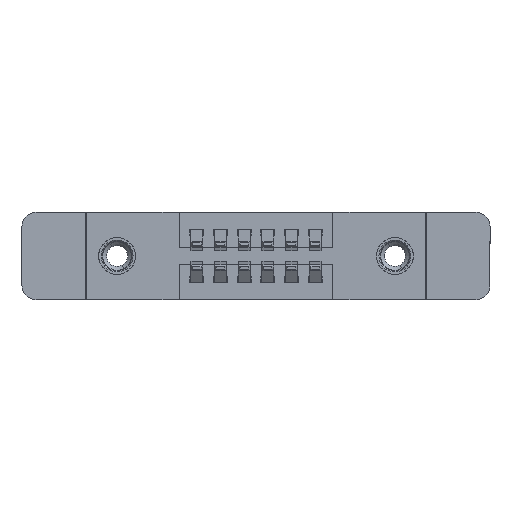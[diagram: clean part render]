
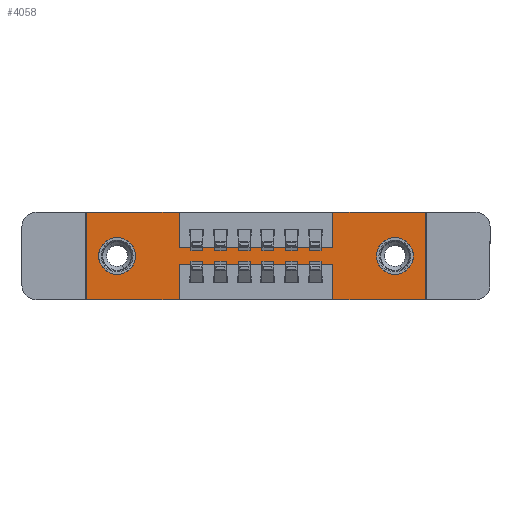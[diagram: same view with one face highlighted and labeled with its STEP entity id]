
A CAD part, front view. The second image highlights one B-rep face of the part: STEP entity #4058.
In plain terms, the highlighted planar face has unit normal (0, -1, 0).
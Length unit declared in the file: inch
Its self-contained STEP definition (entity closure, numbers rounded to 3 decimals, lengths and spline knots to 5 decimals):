
#70 = VECTOR ( 'NONE', #12861, 39.37008 ) ;
#97 = DIRECTION ( 'NONE',  ( 1., 0., 0. ) ) ;
#251 = VECTOR ( 'NONE', #13630, 39.37008 ) ;
#335 = CARTESIAN_POINT ( 'NONE',  ( 0.3925, 0., -0.22 ) ) ;
#415 = CARTESIAN_POINT ( 'NONE',  ( 0., 0., -0.37 ) ) ;
#432 = EDGE_CURVE ( 'NONE', #12691, #13546, #6473, .T. ) ;
#435 = CARTESIAN_POINT ( 'NONE',  ( 1.305, 0., -0.185 ) ) ;
#496 = VERTEX_POINT ( 'NONE', #5100 ) ;
#497 = VERTEX_POINT ( 'NONE', #13150 ) ;
#561 = VECTOR ( 'NONE', #97, 39.37008 ) ;
#679 = ORIENTED_EDGE ( 'NONE', *, *, #7101, .F. ) ;
#723 = ORIENTED_EDGE ( 'NONE', *, *, #10206, .T. ) ;
#831 = CARTESIAN_POINT ( 'NONE',  ( 1.0425, 0., -0.15 ) ) ;
#891 = CIRCLE ( 'NONE', #4677, 0.078 ) ;
#1075 = VECTOR ( 'NONE', #12570, 39.37008 ) ;
#1166 = CARTESIAN_POINT ( 'NONE',  ( 0.3925, 0., -0.15 ) ) ;
#1195 = DIRECTION ( 'NONE',  ( 0., 0., 1. ) ) ;
#1584 = DIRECTION ( 'NONE',  ( 0., 0., -1. ) ) ;
#1616 = DIRECTION ( 'NONE',  ( 0., 0., -1. ) ) ;
#1622 = CARTESIAN_POINT ( 'NONE',  ( 0.3925, 0., -0.15 ) ) ;
#1876 = VECTOR ( 'NONE', #10326, 39.37008 ) ;
#1908 = VERTEX_POINT ( 'NONE', #4619 ) ;
#2002 = ORIENTED_EDGE ( 'NONE', *, *, #9250, .F. ) ;
#2432 = AXIS2_PLACEMENT_3D ( 'NONE', #13286, #6387, #14426 ) ;
#2614 = LINE ( 'NONE', #8051, #5289 ) ;
#2642 = ORIENTED_EDGE ( 'NONE', *, *, #4196, .F. ) ;
#2768 = AXIS2_PLACEMENT_3D ( 'NONE', #435, #8440, #1584 ) ;
#3046 = LINE ( 'NONE', #7247, #8759 ) ;
#3229 = LINE ( 'NONE', #12070, #12024 ) ;
#3339 = CARTESIAN_POINT ( 'NONE',  ( 0., 0., 0. ) ) ;
#3596 = CARTESIAN_POINT ( 'NONE',  ( 1.0425, 0., -0.37 ) ) ;
#3885 = DIRECTION ( 'NONE',  ( -1., 0., 0. ) ) ;
#4048 = VERTEX_POINT ( 'NONE', #4407 ) ;
#4054 = ORIENTED_EDGE ( 'NONE', *, *, #432, .F. ) ;
#4058 = ADVANCED_FACE ( 'NONE', ( #5387, #14192, #11154 ), #12436, .T. ) ;
#4145 = LINE ( 'NONE', #11419, #1075 ) ;
#4196 = EDGE_CURVE ( 'NONE', #5480, #497, #6622, .T. ) ;
#4407 = CARTESIAN_POINT ( 'NONE',  ( 0.3925, 0., -0.22 ) ) ;
#4479 = EDGE_LOOP ( 'NONE', ( #13701, #4687 ) ) ;
#4540 = ORIENTED_EDGE ( 'NONE', *, *, #13030, .F. ) ;
#4611 = VERTEX_POINT ( 'NONE', #6480 ) ;
#4619 = CARTESIAN_POINT ( 'NONE',  ( 0., 0., -0.37 ) ) ;
#4648 = CARTESIAN_POINT ( 'NONE',  ( 0., 0., 0. ) ) ;
#4677 = AXIS2_PLACEMENT_3D ( 'NONE', #13163, #6266, #14307 ) ;
#4687 = ORIENTED_EDGE ( 'NONE', *, *, #11195, .T. ) ;
#4732 = DIRECTION ( 'NONE',  ( 0., 0., 1. ) ) ;
#4754 = CIRCLE ( 'NONE', #2432, 0.078 ) ;
#4905 = LINE ( 'NONE', #12632, #1876 ) ;
#4913 = ORIENTED_EDGE ( 'NONE', *, *, #11304, .F. ) ;
#5100 = CARTESIAN_POINT ( 'NONE',  ( 1.305, 0., -0.263 ) ) ;
#5289 = VECTOR ( 'NONE', #1195, 39.37008 ) ;
#5387 = FACE_BOUND ( 'NONE', #6741, .T. ) ;
#5480 = VERTEX_POINT ( 'NONE', #9616 ) ;
#5573 = CARTESIAN_POINT ( 'NONE',  ( 0., 0., -0.37 ) ) ;
#5585 = DIRECTION ( 'NONE',  ( 0., 1., 0. ) ) ;
#5994 = CARTESIAN_POINT ( 'NONE',  ( 0.13, 0., -0.107 ) ) ;
#6049 = CARTESIAN_POINT ( 'NONE',  ( 1.0425, 0., -0.37 ) ) ;
#6249 = VERTEX_POINT ( 'NONE', #7646 ) ;
#6266 = DIRECTION ( 'NONE',  ( 0., 1., 0. ) ) ;
#6321 = LINE ( 'NONE', #5573, #251 ) ;
#6387 = DIRECTION ( 'NONE',  ( 0., 1., 0. ) ) ;
#6451 = EDGE_LOOP ( 'NONE', ( #7751, #4540, #11044, #4054, #11055, #2642, #679, #9991, #2002, #11478, #4913, #6497 ) ) ;
#6473 = LINE ( 'NONE', #415, #8816 ) ;
#6480 = CARTESIAN_POINT ( 'NONE',  ( 0.3925, 0., -0.37 ) ) ;
#6497 = ORIENTED_EDGE ( 'NONE', *, *, #12739, .F. ) ;
#6622 = LINE ( 'NONE', #4648, #561 ) ;
#6681 = DIRECTION ( 'NONE',  ( 0., -1., 0. ) ) ;
#6741 = EDGE_LOOP ( 'NONE', ( #723, #11023 ) ) ;
#7015 = VERTEX_POINT ( 'NONE', #3339 ) ;
#7067 = CIRCLE ( 'NONE', #12253, 0.078 ) ;
#7101 = EDGE_CURVE ( 'NONE', #7413, #5480, #8811, .T. ) ;
#7247 = CARTESIAN_POINT ( 'NONE',  ( 0.3925, 0., 0. ) ) ;
#7413 = VERTEX_POINT ( 'NONE', #831 ) ;
#7598 = VERTEX_POINT ( 'NONE', #1166 ) ;
#7646 = CARTESIAN_POINT ( 'NONE',  ( 1.0425, 0., -0.22 ) ) ;
#7751 = ORIENTED_EDGE ( 'NONE', *, *, #12359, .F. ) ;
#7804 = EDGE_CURVE ( 'NONE', #7598, #7413, #9677, .T. ) ;
#8051 = CARTESIAN_POINT ( 'NONE',  ( 0., 0., 0. ) ) ;
#8440 = DIRECTION ( 'NONE',  ( 0., 1., 0. ) ) ;
#8685 = EDGE_CURVE ( 'NONE', #7015, #12624, #4145, .T. ) ;
#8759 = VECTOR ( 'NONE', #1616, 39.37008 ) ;
#8811 = LINE ( 'NONE', #11661, #11511 ) ;
#8816 = VECTOR ( 'NONE', #3885, 39.37008 ) ;
#8946 = EDGE_CURVE ( 'NONE', #496, #12266, #891, .T. ) ;
#8972 = EDGE_CURVE ( 'NONE', #497, #12691, #3229, .T. ) ;
#9250 = EDGE_CURVE ( 'NONE', #12624, #7598, #3046, .T. ) ;
#9336 = DIRECTION ( 'NONE',  ( 0., 0., 1. ) ) ;
#9616 = CARTESIAN_POINT ( 'NONE',  ( 1.0425, 0., 0. ) ) ;
#9677 = LINE ( 'NONE', #1622, #12036 ) ;
#9703 = CARTESIAN_POINT ( 'NONE',  ( 0.3925, 0., 0. ) ) ;
#9991 = ORIENTED_EDGE ( 'NONE', *, *, #7804, .F. ) ;
#10206 = EDGE_CURVE ( 'NONE', #12266, #496, #12515, .T. ) ;
#10227 = CARTESIAN_POINT ( 'NONE',  ( 1.305, 0., -0.107 ) ) ;
#10281 = LINE ( 'NONE', #3596, #12980 ) ;
#10326 = DIRECTION ( 'NONE',  ( 0., 0., -1. ) ) ;
#10796 = DIRECTION ( 'NONE',  ( 1., 0., 0. ) ) ;
#10848 = VERTEX_POINT ( 'NONE', #5994 ) ;
#10853 = DIRECTION ( 'NONE',  ( 0., 0., -1. ) ) ;
#11023 = ORIENTED_EDGE ( 'NONE', *, *, #8946, .T. ) ;
#11044 = ORIENTED_EDGE ( 'NONE', *, *, #12943, .F. ) ;
#11055 = ORIENTED_EDGE ( 'NONE', *, *, #8972, .F. ) ;
#11154 = FACE_OUTER_BOUND ( 'NONE', #6451, .T. ) ;
#11195 = EDGE_CURVE ( 'NONE', #12010, #10848, #7067, .T. ) ;
#11275 = AXIS2_PLACEMENT_3D ( 'NONE', #13590, #6681, #14734 ) ;
#11304 = EDGE_CURVE ( 'NONE', #1908, #7015, #2614, .T. ) ;
#11419 = CARTESIAN_POINT ( 'NONE',  ( 0., 0., 0. ) ) ;
#11478 = ORIENTED_EDGE ( 'NONE', *, *, #8685, .F. ) ;
#11511 = VECTOR ( 'NONE', #9336, 39.37008 ) ;
#11661 = CARTESIAN_POINT ( 'NONE',  ( 1.0425, 0., 0. ) ) ;
#11667 = EDGE_CURVE ( 'NONE', #10848, #12010, #4754, .T. ) ;
#11908 = LINE ( 'NONE', #335, #70 ) ;
#11958 = CARTESIAN_POINT ( 'NONE',  ( 0.13, 0., -0.263 ) ) ;
#12010 = VERTEX_POINT ( 'NONE', #11958 ) ;
#12024 = VECTOR ( 'NONE', #10853, 39.37008 ) ;
#12036 = VECTOR ( 'NONE', #10796, 39.37008 ) ;
#12070 = CARTESIAN_POINT ( 'NONE',  ( 1.435, 0., 0. ) ) ;
#12253 = AXIS2_PLACEMENT_3D ( 'NONE', #12488, #5585, #13639 ) ;
#12266 = VERTEX_POINT ( 'NONE', #10227 ) ;
#12359 = EDGE_CURVE ( 'NONE', #4048, #4611, #4905, .T. ) ;
#12436 = PLANE ( 'NONE',  #11275 ) ;
#12488 = CARTESIAN_POINT ( 'NONE',  ( 0.13, 0., -0.185 ) ) ;
#12515 = CIRCLE ( 'NONE', #2768, 0.078 ) ;
#12570 = DIRECTION ( 'NONE',  ( 1., 0., 0. ) ) ;
#12624 = VERTEX_POINT ( 'NONE', #9703 ) ;
#12632 = CARTESIAN_POINT ( 'NONE',  ( 0.3925, 0., -0.37 ) ) ;
#12691 = VERTEX_POINT ( 'NONE', #13495 ) ;
#12739 = EDGE_CURVE ( 'NONE', #4611, #1908, #6321, .T. ) ;
#12861 = DIRECTION ( 'NONE',  ( -1., 0., 0. ) ) ;
#12943 = EDGE_CURVE ( 'NONE', #13546, #6249, #10281, .T. ) ;
#12980 = VECTOR ( 'NONE', #4732, 39.37008 ) ;
#13030 = EDGE_CURVE ( 'NONE', #6249, #4048, #11908, .T. ) ;
#13150 = CARTESIAN_POINT ( 'NONE',  ( 1.435, 0., 0. ) ) ;
#13163 = CARTESIAN_POINT ( 'NONE',  ( 1.305, 0., -0.185 ) ) ;
#13286 = CARTESIAN_POINT ( 'NONE',  ( 0.13, 0., -0.185 ) ) ;
#13495 = CARTESIAN_POINT ( 'NONE',  ( 1.435, 0., -0.37 ) ) ;
#13546 = VERTEX_POINT ( 'NONE', #6049 ) ;
#13590 = CARTESIAN_POINT ( 'NONE',  ( 0., 0., -0.37 ) ) ;
#13630 = DIRECTION ( 'NONE',  ( -1., 0., 0. ) ) ;
#13639 = DIRECTION ( 'NONE',  ( 0., 0., 1. ) ) ;
#13701 = ORIENTED_EDGE ( 'NONE', *, *, #11667, .T. ) ;
#14192 = FACE_BOUND ( 'NONE', #4479, .T. ) ;
#14307 = DIRECTION ( 'NONE',  ( 0., 0., -1. ) ) ;
#14426 = DIRECTION ( 'NONE',  ( 0., 0., 1. ) ) ;
#14734 = DIRECTION ( 'NONE',  ( 0., 0., -1. ) ) ;
